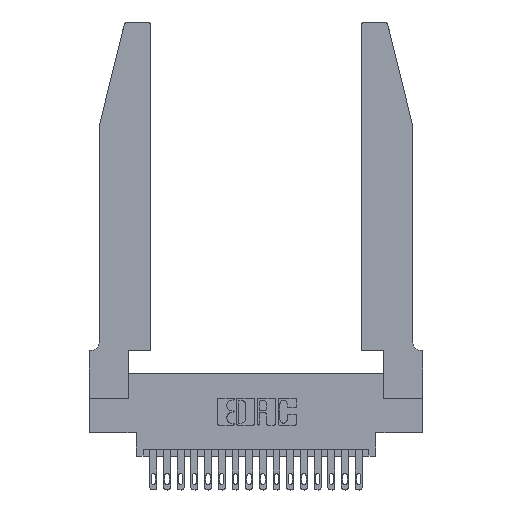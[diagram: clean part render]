
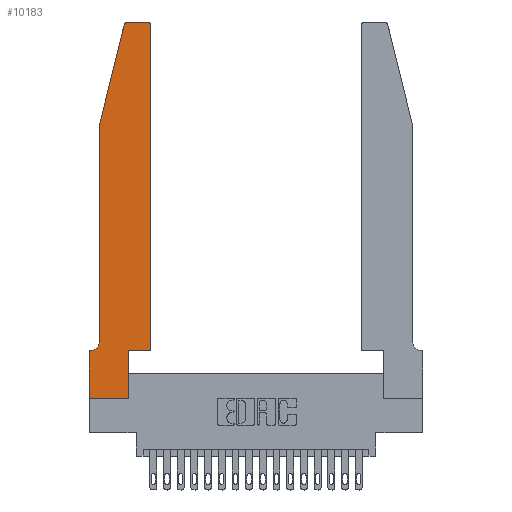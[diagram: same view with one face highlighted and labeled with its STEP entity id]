
A CAD part, top view. The second image highlights one B-rep face of the part: STEP entity #10183.
In plain terms, the highlighted planar face has unit normal (0, 0, 1).
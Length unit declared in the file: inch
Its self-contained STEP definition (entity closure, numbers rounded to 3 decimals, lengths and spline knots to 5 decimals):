
#562 = DIRECTION ( 'NONE',  ( 0., 0., 1. ) ) ;
#1443 = DIRECTION ( 'NONE',  ( 0., 1., 0. ) ) ;
#1588 = EDGE_CURVE ( 'NONE', #1954, #19216, #17977, .T. ) ;
#1696 = DIRECTION ( 'NONE',  ( -1., 0., 0. ) ) ;
#1737 = DIRECTION ( 'NONE',  ( 0., -1., 0. ) ) ;
#1781 = DIRECTION ( 'NONE',  ( 1., 0., 0. ) ) ;
#1903 = VECTOR ( 'NONE', #2496, 39.37008 ) ;
#1954 = VERTEX_POINT ( 'NONE', #13746 ) ;
#2283 = ORIENTED_EDGE ( 'NONE', *, *, #3469, .T. ) ;
#2496 = DIRECTION ( 'NONE',  ( -1., 0., 0. ) ) ;
#3269 = CIRCLE ( 'NONE', #17604, 0.03 ) ;
#3372 = LINE ( 'NONE', #12055, #18797 ) ;
#3404 = DIRECTION ( 'NONE',  ( 0., 0., 1. ) ) ;
#3469 = EDGE_CURVE ( 'NONE', #14414, #4762, #16665, .T. ) ;
#3948 = LINE ( 'NONE', #8882, #1903 ) ;
#3952 = VERTEX_POINT ( 'NONE', #7351 ) ;
#4270 = ORIENTED_EDGE ( 'NONE', *, *, #8067, .T. ) ;
#4271 = CARTESIAN_POINT ( 'NONE',  ( 0.4505, 0.35, 0.37 ) ) ;
#4279 = EDGE_LOOP ( 'NONE', ( #7375, #5120, #6508, #16329, #7847, #9764, #4270, #6075, #18277, #2283, #11288, #16218 ) ) ;
#4417 = EDGE_CURVE ( 'NONE', #14271, #8069, #3269, .T. ) ;
#4487 = LINE ( 'NONE', #6570, #8512 ) ;
#4617 = VECTOR ( 'NONE', #12792, 39.37008 ) ;
#4760 = CARTESIAN_POINT ( 'NONE',  ( 0.4205, 2.75, 0.37 ) ) ;
#4762 = VERTEX_POINT ( 'NONE', #4271 ) ;
#5072 = CARTESIAN_POINT ( 'NONE',  ( 0.2605, 2.75, 0.37 ) ) ;
#5120 = ORIENTED_EDGE ( 'NONE', *, *, #4417, .T. ) ;
#5474 = CARTESIAN_POINT ( 'NONE',  ( 0.25487, 2.72718, 0.37 ) ) ;
#5720 = CARTESIAN_POINT ( 'NONE',  ( 0.2865, 0., 0.37 ) ) ;
#6075 = ORIENTED_EDGE ( 'NONE', *, *, #8914, .T. ) ;
#6103 = LINE ( 'NONE', #11905, #15154 ) ;
#6235 = CARTESIAN_POINT ( 'NONE',  ( 0.0755, 2., 0.37 ) ) ;
#6240 = DIRECTION ( 'NONE',  ( 1., 0., 0. ) ) ;
#6508 = ORIENTED_EDGE ( 'NONE', *, *, #7229, .T. ) ;
#6570 = CARTESIAN_POINT ( 'NONE',  ( 0.0755, 2., 0.37 ) ) ;
#6906 = DIRECTION ( 'NONE',  ( 0., -1., 0. ) ) ;
#7167 = LINE ( 'NONE', #6235, #4617 ) ;
#7229 = EDGE_CURVE ( 'NONE', #8069, #3952, #7167, .T. ) ;
#7351 = CARTESIAN_POINT ( 'NONE',  ( 0.0755, 2., 0.37 ) ) ;
#7375 = ORIENTED_EDGE ( 'NONE', *, *, #11102, .T. ) ;
#7431 = CARTESIAN_POINT ( 'NONE',  ( 0.0055, 0.42, 0.37 ) ) ;
#7847 = ORIENTED_EDGE ( 'NONE', *, *, #1588, .T. ) ;
#8067 = EDGE_CURVE ( 'NONE', #14843, #18218, #6103, .T. ) ;
#8069 = VERTEX_POINT ( 'NONE', #5474 ) ;
#8121 = AXIS2_PLACEMENT_3D ( 'NONE', #7431, #14108, #20368 ) ;
#8512 = VECTOR ( 'NONE', #1737, 39.37008 ) ;
#8621 = CARTESIAN_POINT ( 'NONE',  ( 0., 0.35, 0.37 ) ) ;
#8731 = CARTESIAN_POINT ( 'NONE',  ( 0.0055, 0.35, 0.37 ) ) ;
#8882 = CARTESIAN_POINT ( 'NONE',  ( 0.0755, 0.35, 0.37 ) ) ;
#8914 = EDGE_CURVE ( 'NONE', #18218, #13644, #17146, .T. ) ;
#9361 = VECTOR ( 'NONE', #6240, 39.37008 ) ;
#9599 = EDGE_CURVE ( 'NONE', #9969, #15437, #19131, .T. ) ;
#9764 = ORIENTED_EDGE ( 'NONE', *, *, #12825, .T. ) ;
#9969 = VERTEX_POINT ( 'NONE', #17840 ) ;
#10183 = ADVANCED_FACE ( 'NONE', ( #17353 ), #18108, .T. ) ;
#10185 = DIRECTION ( 'NONE',  ( 1., 0., 0. ) ) ;
#10245 = DIRECTION ( 'NONE',  ( 1., 0., 0. ) ) ;
#10255 = VECTOR ( 'NONE', #1443, 39.37008 ) ;
#10557 = EDGE_CURVE ( 'NONE', #3952, #1954, #4487, .T. ) ;
#11102 = EDGE_CURVE ( 'NONE', #15437, #14271, #12780, .T. ) ;
#11177 = CARTESIAN_POINT ( 'NONE',  ( 0.2865, 0.35, 0.37 ) ) ;
#11288 = ORIENTED_EDGE ( 'NONE', *, *, #11819, .T. ) ;
#11392 = CARTESIAN_POINT ( 'NONE',  ( 0.2865, 0.35, 0.37 ) ) ;
#11661 = CARTESIAN_POINT ( 'NONE',  ( 0., 0., 0.37 ) ) ;
#11819 = EDGE_CURVE ( 'NONE', #4762, #9969, #3372, .T. ) ;
#11905 = CARTESIAN_POINT ( 'NONE',  ( 0., 0., 0.37 ) ) ;
#12055 = CARTESIAN_POINT ( 'NONE',  ( 0.4505, 0.35, 0.37 ) ) ;
#12280 = VECTOR ( 'NONE', #1696, 39.37008 ) ;
#12780 = LINE ( 'NONE', #5072, #12280 ) ;
#12789 = LINE ( 'NONE', #11177, #10255 ) ;
#12792 = DIRECTION ( 'NONE',  ( -0.239, -0.971, 0. ) ) ;
#12825 = EDGE_CURVE ( 'NONE', #19216, #14843, #3948, .T. ) ;
#13052 = EDGE_CURVE ( 'NONE', #13644, #14414, #12789, .T. ) ;
#13381 = CARTESIAN_POINT ( 'NONE',  ( 0.4505, 0.35, 0.37 ) ) ;
#13644 = VERTEX_POINT ( 'NONE', #5720 ) ;
#13746 = CARTESIAN_POINT ( 'NONE',  ( 0.0755, 0.42, 0.37 ) ) ;
#14108 = DIRECTION ( 'NONE',  ( 0., 0., -1. ) ) ;
#14271 = VERTEX_POINT ( 'NONE', #18374 ) ;
#14414 = VERTEX_POINT ( 'NONE', #11392 ) ;
#14647 = VECTOR ( 'NONE', #18186, 39.37008 ) ;
#14843 = VERTEX_POINT ( 'NONE', #18718 ) ;
#15154 = VECTOR ( 'NONE', #6906, 39.37008 ) ;
#15437 = VERTEX_POINT ( 'NONE', #4760 ) ;
#16218 = ORIENTED_EDGE ( 'NONE', *, *, #9599, .T. ) ;
#16307 = CARTESIAN_POINT ( 'NONE',  ( 0.284, 2.72, 0.37 ) ) ;
#16329 = ORIENTED_EDGE ( 'NONE', *, *, #10557, .T. ) ;
#16665 = LINE ( 'NONE', #13381, #14647 ) ;
#16859 = AXIS2_PLACEMENT_3D ( 'NONE', #18197, #562, #10185 ) ;
#17146 = LINE ( 'NONE', #17433, #9361 ) ;
#17353 = FACE_OUTER_BOUND ( 'NONE', #4279, .T. ) ;
#17433 = CARTESIAN_POINT ( 'NONE',  ( 0., 0., 0.37 ) ) ;
#17604 = AXIS2_PLACEMENT_3D ( 'NONE', #16307, #3404, #1781 ) ;
#17840 = CARTESIAN_POINT ( 'NONE',  ( 0.4505, 2.72, 0.37 ) ) ;
#17977 = CIRCLE ( 'NONE', #8121, 0.07 ) ;
#18108 = PLANE ( 'NONE',  #18760 ) ;
#18186 = DIRECTION ( 'NONE',  ( 1., 0., 0. ) ) ;
#18197 = CARTESIAN_POINT ( 'NONE',  ( 0.4205, 2.72, 0.37 ) ) ;
#18218 = VERTEX_POINT ( 'NONE', #11661 ) ;
#18277 = ORIENTED_EDGE ( 'NONE', *, *, #13052, .T. ) ;
#18374 = CARTESIAN_POINT ( 'NONE',  ( 0.284, 2.75, 0.37 ) ) ;
#18589 = DIRECTION ( 'NONE',  ( 0., 1., 0. ) ) ;
#18718 = CARTESIAN_POINT ( 'NONE',  ( 0., 0.35, 0.37 ) ) ;
#18760 = AXIS2_PLACEMENT_3D ( 'NONE', #8621, #20006, #10245 ) ;
#18797 = VECTOR ( 'NONE', #18589, 39.37008 ) ;
#19131 = CIRCLE ( 'NONE', #16859, 0.03 ) ;
#19216 = VERTEX_POINT ( 'NONE', #8731 ) ;
#20006 = DIRECTION ( 'NONE',  ( 0., 0., 1. ) ) ;
#20368 = DIRECTION ( 'NONE',  ( -1., 0., 0. ) ) ;
